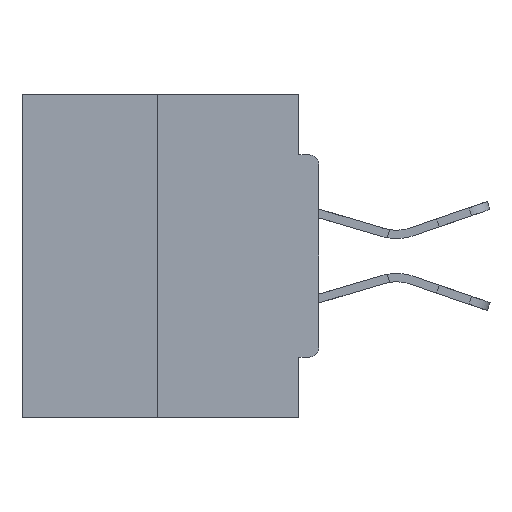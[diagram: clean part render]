
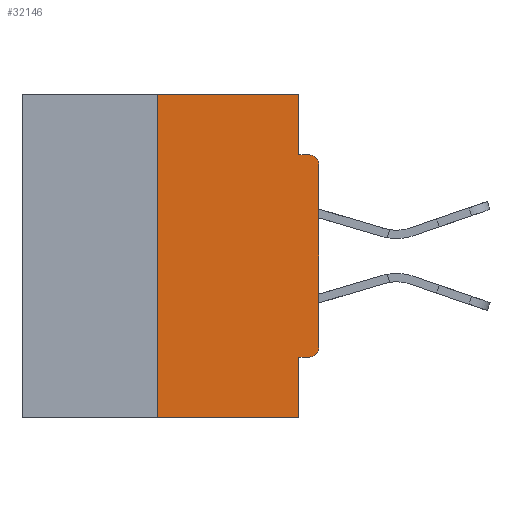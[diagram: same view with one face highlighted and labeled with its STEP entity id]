
A CAD part, left-side view. The second image highlights one B-rep face of the part: STEP entity #32146.
In plain terms, the highlighted planar face has unit normal (-1, 0, 0).
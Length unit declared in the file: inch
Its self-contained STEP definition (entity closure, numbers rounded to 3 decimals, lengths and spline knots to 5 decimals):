
#99 = VERTEX_POINT ( 'NONE', #32690 ) ;
#1312 = VERTEX_POINT ( 'NONE', #17893 ) ;
#1985 = LINE ( 'NONE', #10750, #10864 ) ;
#2058 = CIRCLE ( 'NONE', #22462, 0.015 ) ;
#2625 = CARTESIAN_POINT ( 'NONE',  ( 0., 0.031, 0. ) ) ;
#3425 = DIRECTION ( 'NONE',  ( 0., 0., -1. ) ) ;
#3504 = CARTESIAN_POINT ( 'NONE',  ( 0., 0.015, -0.1085 ) ) ;
#3838 = LINE ( 'NONE', #7182, #13506 ) ;
#3950 = DIRECTION ( 'NONE',  ( 0., 0., -1. ) ) ;
#4170 = CARTESIAN_POINT ( 'NONE',  ( 0., 0.25, 0. ) ) ;
#5344 = EDGE_LOOP ( 'NONE', ( #21810, #11750, #24225, #20303, #29240, #31086, #15747, #23533, #16382, #20496 ) ) ;
#5487 = CARTESIAN_POINT ( 'NONE',  ( 0., 0., -0.1085 ) ) ;
#5743 = VERTEX_POINT ( 'NONE', #15784 ) ;
#6450 = DIRECTION ( 'NONE',  ( -1., 0., 0. ) ) ;
#6995 = CARTESIAN_POINT ( 'NONE',  ( 0., 0.031, 0. ) ) ;
#7077 = CARTESIAN_POINT ( 'NONE',  ( 0., 0.46, 0. ) ) ;
#7182 = CARTESIAN_POINT ( 'NONE',  ( 0., 0., -0.0935 ) ) ;
#7240 = LINE ( 'NONE', #2625, #33229 ) ;
#7314 = CARTESIAN_POINT ( 'NONE',  ( 0., 0.46, -0.5 ) ) ;
#7803 = VECTOR ( 'NONE', #12498, 39.37008 ) ;
#8489 = EDGE_CURVE ( 'NONE', #1312, #14172, #2058, .T. ) ;
#9750 = EDGE_CURVE ( 'NONE', #21094, #17440, #7240, .T. ) ;
#10110 = DIRECTION ( 'NONE',  ( 0., -1., 0. ) ) ;
#10750 = CARTESIAN_POINT ( 'NONE',  ( 0., 0.25, 0. ) ) ;
#10859 = DIRECTION ( 'NONE',  ( 0., 0., 1. ) ) ;
#10864 = VECTOR ( 'NONE', #10859, 39.37008 ) ;
#10992 = VECTOR ( 'NONE', #12675, 39.37008 ) ;
#11502 = VERTEX_POINT ( 'NONE', #26371 ) ;
#11750 = ORIENTED_EDGE ( 'NONE', *, *, #31512, .F. ) ;
#11989 = CARTESIAN_POINT ( 'NONE',  ( 0., 0., -0.4065 ) ) ;
#12498 = DIRECTION ( 'NONE',  ( 0., 0., 1. ) ) ;
#12534 = EDGE_CURVE ( 'NONE', #11502, #5743, #16801, .T. ) ;
#12618 = EDGE_CURVE ( 'NONE', #17440, #31431, #3838, .T. ) ;
#12675 = DIRECTION ( 'NONE',  ( 0., -1., 0. ) ) ;
#13008 = CARTESIAN_POINT ( 'NONE',  ( 0., 0.015, -0.0935 ) ) ;
#13506 = VECTOR ( 'NONE', #10110, 39.37008 ) ;
#13683 = EDGE_CURVE ( 'NONE', #14172, #25913, #32164, .T. ) ;
#14172 = VERTEX_POINT ( 'NONE', #25803 ) ;
#15047 = AXIS2_PLACEMENT_3D ( 'NONE', #7077, #25205, #30466 ) ;
#15063 = DIRECTION ( 'NONE',  ( 0., 0., -1. ) ) ;
#15480 = AXIS2_PLACEMENT_3D ( 'NONE', #3504, #6450, #3950 ) ;
#15747 = ORIENTED_EDGE ( 'NONE', *, *, #13683, .T. ) ;
#15784 = CARTESIAN_POINT ( 'NONE',  ( 0., 0.031, -0.5 ) ) ;
#16267 = EDGE_CURVE ( 'NONE', #22367, #21094, #21898, .T. ) ;
#16331 = DIRECTION ( 'NONE',  ( -1., 0., 0. ) ) ;
#16382 = ORIENTED_EDGE ( 'NONE', *, *, #12618, .F. ) ;
#16801 = LINE ( 'NONE', #33175, #28207 ) ;
#17440 = VERTEX_POINT ( 'NONE', #29649 ) ;
#17893 = CARTESIAN_POINT ( 'NONE',  ( 0., 0.015, -0.4065 ) ) ;
#18134 = FACE_OUTER_BOUND ( 'NONE', #5344, .T. ) ;
#18652 = EDGE_CURVE ( 'NONE', #1312, #11502, #23370, .T. ) ;
#19853 = VECTOR ( 'NONE', #32083, 39.37008 ) ;
#20303 = ORIENTED_EDGE ( 'NONE', *, *, #12534, .F. ) ;
#20496 = ORIENTED_EDGE ( 'NONE', *, *, #9750, .F. ) ;
#20567 = CARTESIAN_POINT ( 'NONE',  ( 0., 0.015, -0.3915 ) ) ;
#20681 = DIRECTION ( 'NONE',  ( 0., 0., -1. ) ) ;
#21094 = VERTEX_POINT ( 'NONE', #6995 ) ;
#21554 = LINE ( 'NONE', #7314, #10992 ) ;
#21810 = ORIENTED_EDGE ( 'NONE', *, *, #16267, .F. ) ;
#21898 = LINE ( 'NONE', #31963, #19853 ) ;
#22316 = EDGE_CURVE ( 'NONE', #25913, #31431, #24264, .T. ) ;
#22367 = VERTEX_POINT ( 'NONE', #4170 ) ;
#22462 = AXIS2_PLACEMENT_3D ( 'NONE', #20567, #16331, #20681 ) ;
#22868 = CARTESIAN_POINT ( 'NONE',  ( 0., 0., 0. ) ) ;
#23370 = LINE ( 'NONE', #11989, #23769 ) ;
#23533 = ORIENTED_EDGE ( 'NONE', *, *, #22316, .T. ) ;
#23769 = VECTOR ( 'NONE', #24765, 39.37008 ) ;
#24225 = ORIENTED_EDGE ( 'NONE', *, *, #30011, .T. ) ;
#24264 = CIRCLE ( 'NONE', #15480, 0.015 ) ;
#24765 = DIRECTION ( 'NONE',  ( 0., 1., 0. ) ) ;
#25205 = DIRECTION ( 'NONE',  ( 1., 0., 0. ) ) ;
#25803 = CARTESIAN_POINT ( 'NONE',  ( 0., 0., -0.3915 ) ) ;
#25913 = VERTEX_POINT ( 'NONE', #5487 ) ;
#26371 = CARTESIAN_POINT ( 'NONE',  ( 0., 0.031, -0.4065 ) ) ;
#27972 = PLANE ( 'NONE',  #15047 ) ;
#28207 = VECTOR ( 'NONE', #15063, 39.37008 ) ;
#29240 = ORIENTED_EDGE ( 'NONE', *, *, #18652, .F. ) ;
#29649 = CARTESIAN_POINT ( 'NONE',  ( 0., 0.031, -0.0935 ) ) ;
#30011 = EDGE_CURVE ( 'NONE', #99, #5743, #21554, .T. ) ;
#30466 = DIRECTION ( 'NONE',  ( 0., 0., -1. ) ) ;
#31086 = ORIENTED_EDGE ( 'NONE', *, *, #8489, .T. ) ;
#31431 = VERTEX_POINT ( 'NONE', #13008 ) ;
#31512 = EDGE_CURVE ( 'NONE', #99, #22367, #1985, .T. ) ;
#31963 = CARTESIAN_POINT ( 'NONE',  ( 0., 0.46, 0. ) ) ;
#32083 = DIRECTION ( 'NONE',  ( 0., -1., 0. ) ) ;
#32146 = ADVANCED_FACE ( 'NONE', ( #18134 ), #27972, .F. ) ;
#32164 = LINE ( 'NONE', #22868, #7803 ) ;
#32690 = CARTESIAN_POINT ( 'NONE',  ( 0., 0.25, -0.5 ) ) ;
#33175 = CARTESIAN_POINT ( 'NONE',  ( 0., 0.031, -0.5 ) ) ;
#33229 = VECTOR ( 'NONE', #3425, 39.37008 ) ;
